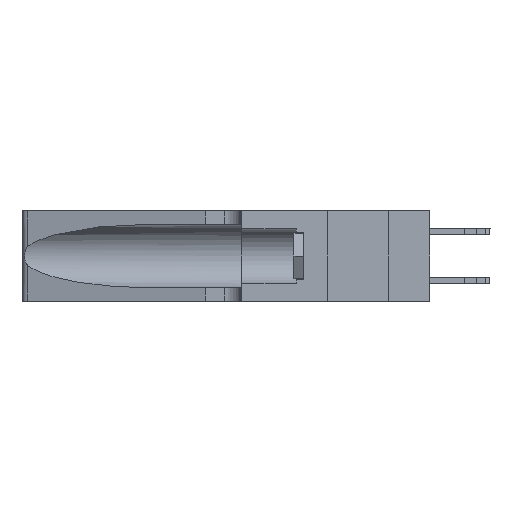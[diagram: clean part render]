
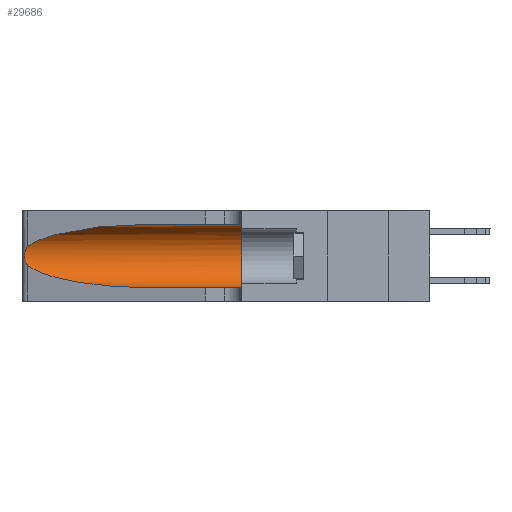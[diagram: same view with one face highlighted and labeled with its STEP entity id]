
A CAD part, left-side view. The second image highlights one B-rep face of the part: STEP entity #29686.
In plain terms, the highlighted cylindrical face has radius 3.308 mm (diameter 6.617 mm), a partial arc.
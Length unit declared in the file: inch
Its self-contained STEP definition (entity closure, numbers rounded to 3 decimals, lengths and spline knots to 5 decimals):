
#315 = VERTEX_POINT ( 'NONE', #4371 ) ;
#1194 = EDGE_CURVE ( 'NONE', #18494, #33330, #3315, .T. ) ;
#1561 = CARTESIAN_POINT ( 'NONE',  ( 0.25856, 1.23593, 0.16098 ) ) ;
#2331 = CARTESIAN_POINT ( 'NONE',  ( 0.25639, 1.23186, 0.15144 ) ) ;
#2623 = CARTESIAN_POINT ( 'NONE',  ( 0.1305, 1.61858, 0.05475 ) ) ;
#3093 = FACE_OUTER_BOUND ( 'NONE', #4258, .T. ) ;
#3315 = CIRCLE ( 'NONE', #14433, 0.13025 ) ;
#3518 = LINE ( 'NONE', #14209, #6141 ) ;
#4258 = EDGE_LOOP ( 'NONE', ( #8085, #35002, #14809, #14805, #24402, #34588 ) ) ;
#4371 = CARTESIAN_POINT ( 'NONE',  ( 0.25487, 1.22718, 0.14631 ) ) ;
#4527 = DIRECTION ( 'NONE',  ( 0., 0., -1. ) ) ;
#5949 = VERTEX_POINT ( 'NONE', #32576 ) ;
#6141 = VECTOR ( 'NONE', #30968, 39.37008 ) ;
#6476 = CARTESIAN_POINT ( 'NONE',  ( 0.1305, 0.72297, 0.05475 ) ) ;
#6514 = EDGE_CURVE ( 'NONE', #5949, #10603, #32693, .T. ) ;
#6861 = CARTESIAN_POINT ( 'NONE',  ( 0.1305, 1.61858, 0.185 ) ) ;
#7643 = EDGE_CURVE ( 'NONE', #10603, #315, #11279, .T. ) ;
#8085 = ORIENTED_EDGE ( 'NONE', *, *, #6514, .T. ) ;
#8137 = CARTESIAN_POINT ( 'NONE',  ( 0.25787, 1.23484, 0.2124 ) ) ;
#8264 = CARTESIAN_POINT ( 'NONE',  ( 0.25555, 1.22994, 0.2215 ) ) ;
#8297 = CARTESIAN_POINT ( 'NONE',  ( 0.18966, 0.96281, 0.05475 ) ) ;
#8406 = CARTESIAN_POINT ( 'NONE',  ( 0.2373, 1.15595, 0.08982 ) ) ;
#8579 = CARTESIAN_POINT ( 'NONE',  ( 0.25555, 1.22993, 0.14849 ) ) ;
#8852 = AXIS2_PLACEMENT_3D ( 'NONE', #6861, #29179, #4527 ) ;
#9268 = CARTESIAN_POINT ( 'NONE',  ( 0.1305, 0.72297, 0.31525 ) ) ;
#10603 = VERTEX_POINT ( 'NONE', #31914 ) ;
#11106 = CARTESIAN_POINT ( 'NONE',  ( 0.25639, 1.23184, 0.21858 ) ) ;
#11279 = B_SPLINE_CURVE_WITH_KNOTS ( 'NONE', 3,
 ( #13282, #8264, #11106, #8137, #35621, #12324, #15742, #28193, #31378, #1561, #30320, #2331, #8579, #27610 ),
 .UNSPECIFIED., .F., .F.,
 ( 4, 2, 2, 2, 2, 2, 4 ),
 ( 0., 0.00027, 0.00053, 0.00107, 0.0016, 0.00187, 0.00214 ),
 .UNSPECIFIED. ) ;
#12324 = CARTESIAN_POINT ( 'NONE',  ( 0.26018, 1.23835, 0.19895 ) ) ;
#12417 = EDGE_CURVE ( 'NONE', #5949, #18494, #3518, .T. ) ;
#12485 = CARTESIAN_POINT ( 'NONE',  ( 0.18966, 0.96281, 0.31525 ) ) ;
#13282 = CARTESIAN_POINT ( 'NONE',  ( 0.25487, 1.22718, 0.22369 ) ) ;
#13815 = VECTOR ( 'NONE', #25175, 39.37008 ) ;
#14209 = CARTESIAN_POINT ( 'NONE',  ( 0.1305, 1.61858, 0.31525 ) ) ;
#14433 = AXIS2_PLACEMENT_3D ( 'NONE', #19549, #25663, #22714 ) ;
#14805 = ORIENTED_EDGE ( 'NONE', *, *, #21265, .T. ) ;
#14809 = ORIENTED_EDGE ( 'NONE', *, *, #35663, .T. ) ;
#15742 = CARTESIAN_POINT ( 'NONE',  ( 0.26075, 1.23896, 0.19203 ) ) ;
#16854 = CYLINDRICAL_SURFACE ( 'NONE', #8852, 0.13025 ) ;
#18193 = LINE ( 'NONE', #2623, #13815 ) ;
#18494 = VERTEX_POINT ( 'NONE', #29793 ) ;
#19549 = CARTESIAN_POINT ( 'NONE',  ( 0.1305, 0.35, 0.185 ) ) ;
#20453 = CARTESIAN_POINT ( 'NONE',  ( 0.2373, 1.15595, 0.28018 ) ) ;
#21265 = EDGE_CURVE ( 'NONE', #29658, #33330, #18193, .T. ) ;
#22207 = CARTESIAN_POINT ( 'NONE',  ( 0.25487, 1.22718, 0.14631 ) ) ;
#22714 = DIRECTION ( 'NONE',  ( 0., 0., 1. ) ) ;
#23312 = CARTESIAN_POINT ( 'NONE',  ( 0.1305, 0.35, 0.05475 ) ) ;
#24402 = ORIENTED_EDGE ( 'NONE', *, *, #1194, .F. ) ;
#25175 = DIRECTION ( 'NONE',  ( 0., -1., 0. ) ) ;
#25663 = DIRECTION ( 'NONE',  ( 0., 1., 0. ) ) ;
#27610 = CARTESIAN_POINT ( 'NONE',  ( 0.25487, 1.22718, 0.14631 ) ) ;
#27893 = CARTESIAN_POINT ( 'NONE',  ( 0.1305, 0.72297, 0.05475 ) ) ;
#28193 = CARTESIAN_POINT ( 'NONE',  ( 0.26075, 1.23896, 0.178 ) ) ;
#28973 = CARTESIAN_POINT ( 'NONE',  ( 0.25487, 1.22718, 0.22369 ) ) ;
#29179 = DIRECTION ( 'NONE',  ( 0., -1., 0. ) ) ;
#29658 = VERTEX_POINT ( 'NONE', #6476 ) ;
#29686 = ADVANCED_FACE ( 'NONE', ( #3093 ), #16854, .F. ) ;
#29793 = CARTESIAN_POINT ( 'NONE',  ( 0.1305, 0.35, 0.31525 ) ) ;
#30320 = CARTESIAN_POINT ( 'NONE',  ( 0.25789, 1.23486, 0.15765 ) ) ;
#30968 = DIRECTION ( 'NONE',  ( 0., -1., 0. ) ) ;
#31378 = CARTESIAN_POINT ( 'NONE',  ( 0.26017, 1.23833, 0.17102 ) ) ;
#31529 =( BOUNDED_CURVE ( )  B_SPLINE_CURVE ( 3, ( #22207, #8406, #8297, #27893 ),
 .UNSPECIFIED., .F., .F. ) 
 B_SPLINE_CURVE_WITH_KNOTS ( ( 4, 4 ),
 ( 3.44316, 4.71239 ),
 .UNSPECIFIED. ) 
 CURVE ( )  GEOMETRIC_REPRESENTATION_ITEM ( )  RATIONAL_B_SPLINE_CURVE ( ( 1., 0.87, 0.87, 1. ) ) 
 REPRESENTATION_ITEM ( '' )  );
#31914 = CARTESIAN_POINT ( 'NONE',  ( 0.25487, 1.22718, 0.22369 ) ) ;
#32576 = CARTESIAN_POINT ( 'NONE',  ( 0.1305, 0.72297, 0.31525 ) ) ;
#32693 =( BOUNDED_CURVE ( )  B_SPLINE_CURVE ( 3, ( #9268, #12485, #20453, #28973 ),
 .UNSPECIFIED., .F., .F. ) 
 B_SPLINE_CURVE_WITH_KNOTS ( ( 4, 4 ),
 ( 1.5708, 2.84003 ),
 .UNSPECIFIED. ) 
 CURVE ( )  GEOMETRIC_REPRESENTATION_ITEM ( )  RATIONAL_B_SPLINE_CURVE ( ( 1., 0.87, 0.87, 1. ) ) 
 REPRESENTATION_ITEM ( '' )  );
#33330 = VERTEX_POINT ( 'NONE', #23312 ) ;
#34588 = ORIENTED_EDGE ( 'NONE', *, *, #12417, .F. ) ;
#35002 = ORIENTED_EDGE ( 'NONE', *, *, #7643, .T. ) ;
#35621 = CARTESIAN_POINT ( 'NONE',  ( 0.25854, 1.2359, 0.20912 ) ) ;
#35663 = EDGE_CURVE ( 'NONE', #315, #29658, #31529, .T. ) ;
